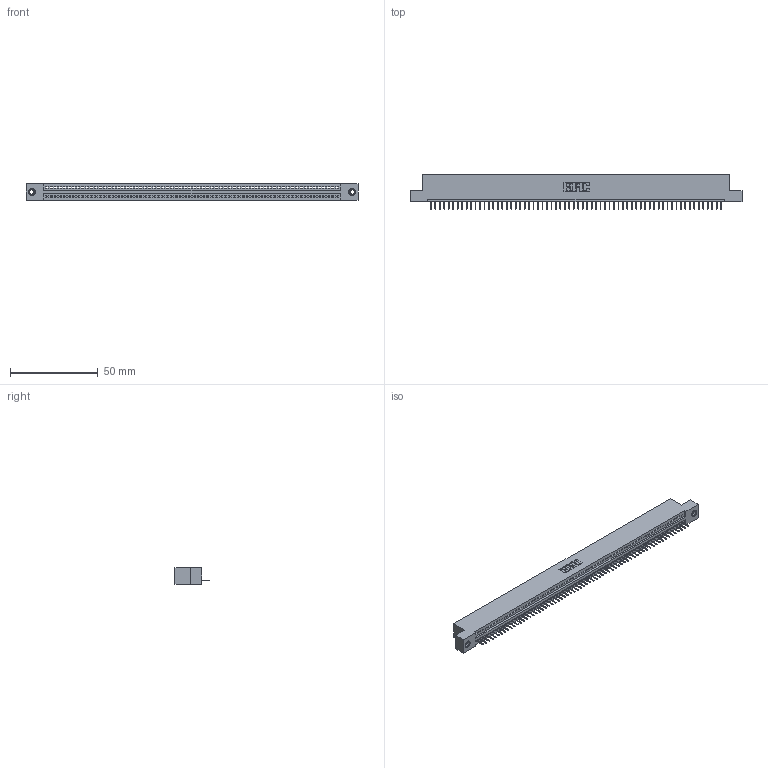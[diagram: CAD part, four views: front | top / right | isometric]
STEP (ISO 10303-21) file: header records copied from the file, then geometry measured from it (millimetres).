
FILE_DESCRIPTION (( 'STEP AP203' ), '1' );
FILE_NAME ('345-066-524-107.STEP', '2018-09-28T20:10:32', ( '' ), ( '' ), 'SwSTEP 2.0', 'SolidWorks 2016', '' );
FILE_SCHEMA (( 'CONFIG_CONTROL_DESIGN' ));
Length unit declared in the file: inch
Products named in the file (4): 345-250-001_345-250-005-103; 345 Part_Flush Mounting Lugs - 0.156 Dia-TI; 345-292-001_345-293-124; 345-066-524-107
Assembly tree (69 placements, depth 2):
  345-066-524-107
    345 Part_Flush Mounting Lugs - 0.156 Dia-TI
    345-292-001_345-293-124  x66
    345-250-001_345-250-005-103  x2
Bounding box: 188.85 x 19.35 x 9.4 mm (x, y, z)
Volume: 17859.4 mm3; surface area: 23258.7 mm2
Topology: 69 solids, 69 shells, 4278 faces, 12357 edges, 7966 vertices
Faces by surface type: plane 3148, cylinder 1114, cone 12, torus 4
Entity records: 47702 total; most frequent: CARTESIAN_POINT 8241, ORIENTED_EDGE 8234, DIRECTION 7191, EDGE_CURVE 4117, VECTOR 3705, LINE 3705, VERTEX_POINT 2736, AXIS2_PLACEMENT_3D 1743
